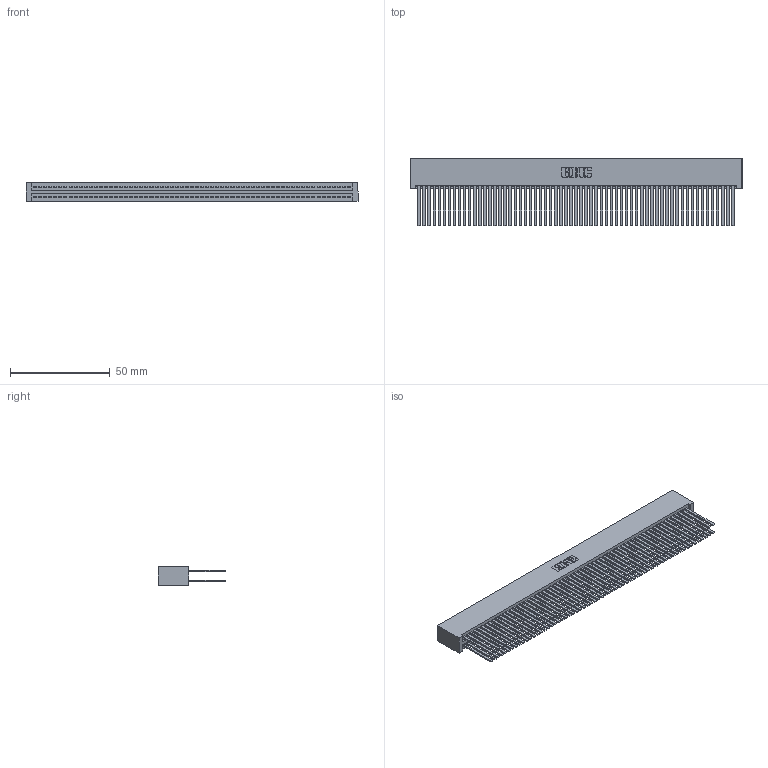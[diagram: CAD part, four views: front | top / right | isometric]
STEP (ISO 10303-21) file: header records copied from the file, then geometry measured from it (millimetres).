
FILE_DESCRIPTION (( 'STEP AP203' ), '1' );
FILE_NAME ('345-126-544-201.STEP', '2019-11-07T04:35:01', ( '' ), ( '' ), 'SwSTEP 2.0', 'SolidWorks 2016', '' );
FILE_SCHEMA (( 'CONFIG_CONTROL_DESIGN' ));
Length unit declared in the file: inch
Products named in the file (3): 345-126-544-201; 345 Part_No Mounting Lugs; 345-292-001_345-293-144
Assembly tree (127 placements, depth 2):
  345-126-544-201
    345 Part_No Mounting Lugs
    345-292-001_345-293-144  x126
Bounding box: 166.62 x 33.96 x 9.4 mm (x, y, z)
Volume: 18763.1 mm3; surface area: 33621.9 mm2
Topology: 127 solids, 127 shells, 5662 faces, 16823 edges, 11046 vertices
Faces by surface type: plane 3730, cylinder 1932
Entity records: 46143 total; most frequent: CARTESIAN_POINT 7712, ORIENTED_EDGE 7646, DIRECTION 6767, EDGE_CURVE 3823, VECTOR 3451, LINE 3451, VERTEX_POINT 2546, AXIS2_PLACEMENT_3D 1658
